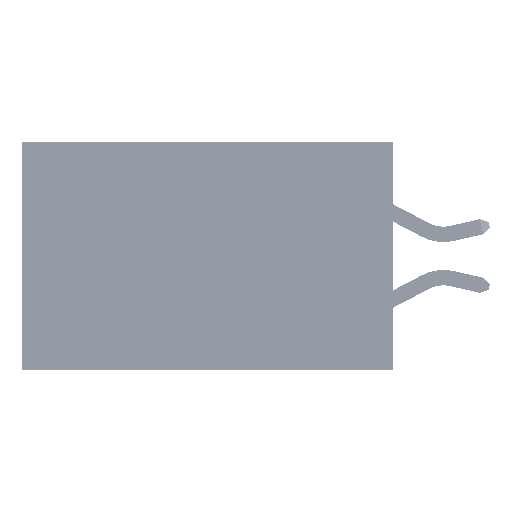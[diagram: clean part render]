
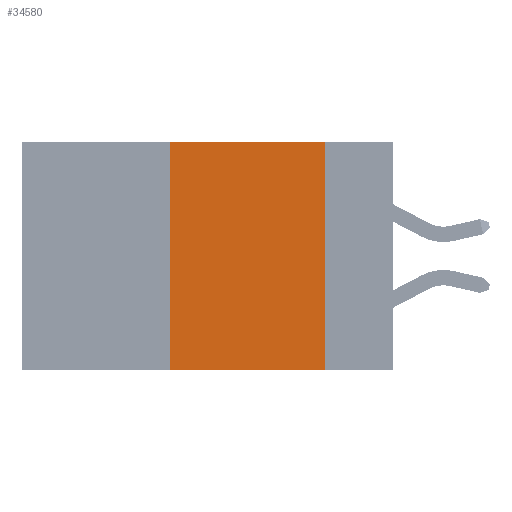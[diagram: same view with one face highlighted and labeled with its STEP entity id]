
A CAD part, left-side view. The second image highlights one B-rep face of the part: STEP entity #34580.
In plain terms, the highlighted planar face has unit normal (-1, 0, 0).
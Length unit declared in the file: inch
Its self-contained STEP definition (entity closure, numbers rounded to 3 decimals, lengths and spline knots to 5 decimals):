
#830 = ORIENTED_EDGE ( 'NONE', *, *, #27708, .F. ) ;
#1873 = FACE_OUTER_BOUND ( 'NONE', #22160, .T. ) ;
#3438 = CARTESIAN_POINT ( 'NONE',  ( 0., 0.6, 0. ) ) ;
#4924 = CARTESIAN_POINT ( 'NONE',  ( 0., 0.11, 0. ) ) ;
#6329 = EDGE_CURVE ( 'NONE', #15967, #19316, #31110, .T. ) ;
#8228 = DIRECTION ( 'NONE',  ( 0., 0., -1. ) ) ;
#11695 = LINE ( 'NONE', #33529, #19778 ) ;
#15119 = ORIENTED_EDGE ( 'NONE', *, *, #22858, .T. ) ;
#15967 = VERTEX_POINT ( 'NONE', #45653 ) ;
#16186 = CARTESIAN_POINT ( 'NONE',  ( 0., 0.11, -0.37 ) ) ;
#16407 = LINE ( 'NONE', #4924, #48091 ) ;
#18390 = VECTOR ( 'NONE', #39606, 39.37008 ) ;
#19226 = CARTESIAN_POINT ( 'NONE',  ( 0., 0.36, 0. ) ) ;
#19316 = VERTEX_POINT ( 'NONE', #33569 ) ;
#19778 = VECTOR ( 'NONE', #42392, 39.37008 ) ;
#20570 = VECTOR ( 'NONE', #39142, 39.37008 ) ;
#22160 = EDGE_LOOP ( 'NONE', ( #49171, #830, #36078, #15119 ) ) ;
#22858 = EDGE_CURVE ( 'NONE', #15967, #41919, #28903, .T. ) ;
#24398 = EDGE_CURVE ( 'NONE', #45802, #41919, #16407, .T. ) ;
#26055 = CARTESIAN_POINT ( 'NONE',  ( 0., 0.11, 0. ) ) ;
#27708 = EDGE_CURVE ( 'NONE', #19316, #45802, #11695, .T. ) ;
#28903 = LINE ( 'NONE', #51155, #18390 ) ;
#31110 = LINE ( 'NONE', #19226, #20570 ) ;
#31393 = DIRECTION ( 'NONE',  ( 1., 0., 0. ) ) ;
#33529 = CARTESIAN_POINT ( 'NONE',  ( 0., 0.6, 0. ) ) ;
#33569 = CARTESIAN_POINT ( 'NONE',  ( 0., 0.36, 0. ) ) ;
#34580 = ADVANCED_FACE ( 'NONE', ( #1873 ), #42542, .F. ) ;
#36078 = ORIENTED_EDGE ( 'NONE', *, *, #6329, .F. ) ;
#39142 = DIRECTION ( 'NONE',  ( 0., 0., 1. ) ) ;
#39606 = DIRECTION ( 'NONE',  ( 0., -1., 0. ) ) ;
#41919 = VERTEX_POINT ( 'NONE', #16186 ) ;
#42392 = DIRECTION ( 'NONE',  ( 0., -1., 0. ) ) ;
#42542 = PLANE ( 'NONE',  #44222 ) ;
#44222 = AXIS2_PLACEMENT_3D ( 'NONE', #3438, #31393, #51278 ) ;
#45653 = CARTESIAN_POINT ( 'NONE',  ( 0., 0.36, -0.37 ) ) ;
#45802 = VERTEX_POINT ( 'NONE', #26055 ) ;
#48091 = VECTOR ( 'NONE', #8228, 39.37008 ) ;
#49171 = ORIENTED_EDGE ( 'NONE', *, *, #24398, .F. ) ;
#51155 = CARTESIAN_POINT ( 'NONE',  ( 0., 0.6, -0.37 ) ) ;
#51278 = DIRECTION ( 'NONE',  ( 0., 0., -1. ) ) ;
